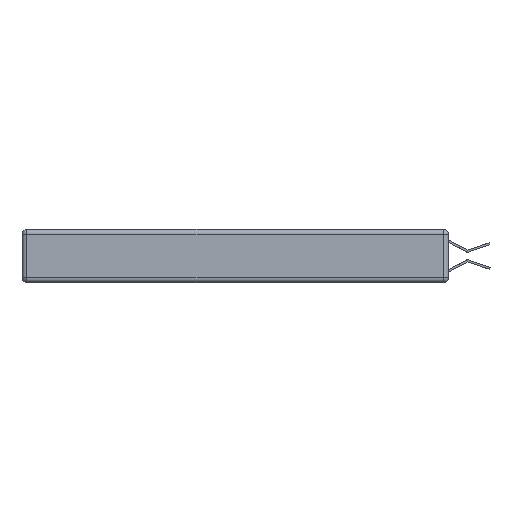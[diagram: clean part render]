
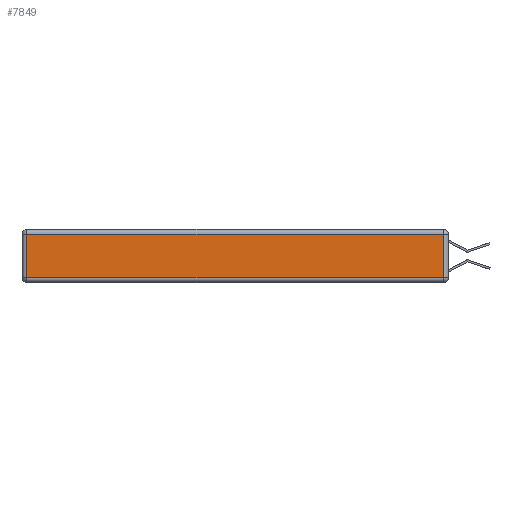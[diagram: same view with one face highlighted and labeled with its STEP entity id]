
A CAD part, left-side view. The second image highlights one B-rep face of the part: STEP entity #7849.
In plain terms, the highlighted planar face has unit normal (-1, 0, 0).
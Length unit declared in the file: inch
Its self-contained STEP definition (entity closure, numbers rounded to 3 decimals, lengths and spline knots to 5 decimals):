
#8 = AXIS2_PLACEMENT_3D ( 'NONE', #11024, #1960, #7796 ) ;
#772 = EDGE_CURVE ( 'NONE', #11988, #10036, #4090, .T. ) ;
#1343 = EDGE_CURVE ( 'NONE', #8887, #11988, #9437, .T. ) ;
#1421 = ORIENTED_EDGE ( 'NONE', *, *, #11144, .T. ) ;
#1575 = VECTOR ( 'NONE', #12131, 39.37008 ) ;
#1857 = VECTOR ( 'NONE', #9846, 39.37008 ) ;
#1960 = DIRECTION ( 'NONE',  ( -1., 0., 0. ) ) ;
#2071 = CARTESIAN_POINT ( 'NONE',  ( 0., 0.03, -0.343 ) ) ;
#2102 = VERTEX_POINT ( 'NONE', #4859 ) ;
#2355 = DIRECTION ( 'NONE',  ( 0., 1., 0. ) ) ;
#4090 = LINE ( 'NONE', #10005, #4686 ) ;
#4605 = CARTESIAN_POINT ( 'NONE',  ( 0., 0.03, -0.03 ) ) ;
#4644 = ORIENTED_EDGE ( 'NONE', *, *, #772, .T. ) ;
#4686 = VECTOR ( 'NONE', #13039, 39.37008 ) ;
#4859 = CARTESIAN_POINT ( 'NONE',  ( 0., 0.03, -0.313 ) ) ;
#5215 = EDGE_CURVE ( 'NONE', #10036, #2102, #7675, .T. ) ;
#5591 = ORIENTED_EDGE ( 'NONE', *, *, #1343, .T. ) ;
#6785 = ORIENTED_EDGE ( 'NONE', *, *, #5215, .T. ) ;
#7013 = FACE_OUTER_BOUND ( 'NONE', #8710, .T. ) ;
#7126 = LINE ( 'NONE', #2071, #1575 ) ;
#7633 = CARTESIAN_POINT ( 'NONE',  ( 0., 2.72, -0.03 ) ) ;
#7675 = LINE ( 'NONE', #11944, #1857 ) ;
#7739 = VECTOR ( 'NONE', #2355, 39.37008 ) ;
#7770 = CARTESIAN_POINT ( 'NONE',  ( 0., 2.72, -0.313 ) ) ;
#7796 = DIRECTION ( 'NONE',  ( 0., 0., 1. ) ) ;
#7849 = ADVANCED_FACE ( 'NONE', ( #7013 ), #11092, .T. ) ;
#8710 = EDGE_LOOP ( 'NONE', ( #6785, #1421, #5591, #4644 ) ) ;
#8887 = VERTEX_POINT ( 'NONE', #4605 ) ;
#9437 = LINE ( 'NONE', #11414, #7739 ) ;
#9846 = DIRECTION ( 'NONE',  ( 0., -1., 0. ) ) ;
#10005 = CARTESIAN_POINT ( 'NONE',  ( 0., 2.72, -0.343 ) ) ;
#10036 = VERTEX_POINT ( 'NONE', #7770 ) ;
#11024 = CARTESIAN_POINT ( 'NONE',  ( 0., 0., -0.343 ) ) ;
#11092 = PLANE ( 'NONE',  #8 ) ;
#11144 = EDGE_CURVE ( 'NONE', #2102, #8887, #7126, .T. ) ;
#11414 = CARTESIAN_POINT ( 'NONE',  ( 0., 2.75, -0.03 ) ) ;
#11944 = CARTESIAN_POINT ( 'NONE',  ( 0., 0., -0.313 ) ) ;
#11988 = VERTEX_POINT ( 'NONE', #7633 ) ;
#12131 = DIRECTION ( 'NONE',  ( 0., 0., 1. ) ) ;
#13039 = DIRECTION ( 'NONE',  ( 0., 0., -1. ) ) ;
